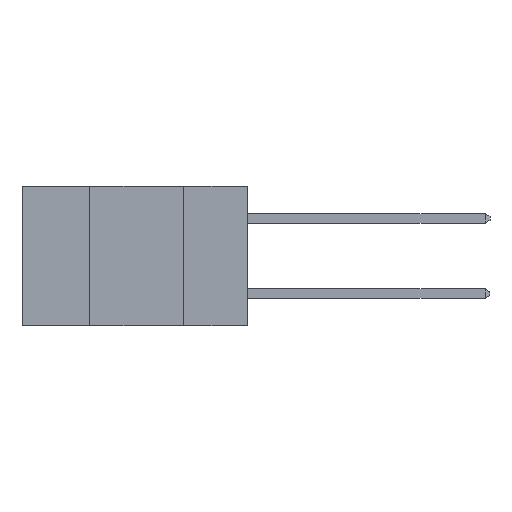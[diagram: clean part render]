
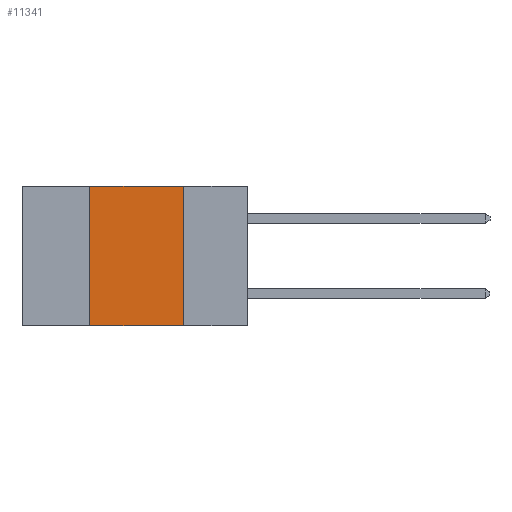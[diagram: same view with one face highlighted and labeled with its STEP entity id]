
A CAD part, left-side view. The second image highlights one B-rep face of the part: STEP entity #11341.
In plain terms, the highlighted planar face has unit normal (-1, 0, 0).
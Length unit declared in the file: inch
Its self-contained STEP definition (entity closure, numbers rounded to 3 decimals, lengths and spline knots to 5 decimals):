
#342 = VECTOR ( 'NONE', #9666, 39.37008 ) ;
#1164 = CARTESIAN_POINT ( 'NONE',  ( 0., 0.42, 0. ) ) ;
#1692 = CARTESIAN_POINT ( 'NONE',  ( 0., 0.6, -0.37 ) ) ;
#2035 = ORIENTED_EDGE ( 'NONE', *, *, #3957, .F. ) ;
#2105 = ORIENTED_EDGE ( 'NONE', *, *, #18469, .F. ) ;
#2183 = CARTESIAN_POINT ( 'NONE',  ( 0., 0.42, -0.37 ) ) ;
#2289 = LINE ( 'NONE', #7527, #10211 ) ;
#2621 = CARTESIAN_POINT ( 'NONE',  ( 0., 0.42, 0. ) ) ;
#2754 = ORIENTED_EDGE ( 'NONE', *, *, #2788, .F. ) ;
#2788 = EDGE_CURVE ( 'NONE', #3424, #3328, #13982, .T. ) ;
#3208 = CARTESIAN_POINT ( 'NONE',  ( 0., 0.6, 0. ) ) ;
#3328 = VERTEX_POINT ( 'NONE', #1164 ) ;
#3424 = VERTEX_POINT ( 'NONE', #2183 ) ;
#3551 = ORIENTED_EDGE ( 'NONE', *, *, #16769, .T. ) ;
#3810 = CARTESIAN_POINT ( 'NONE',  ( 0., 0.6, 0. ) ) ;
#3957 = EDGE_CURVE ( 'NONE', #9337, #6340, #2289, .T. ) ;
#4286 = DIRECTION ( 'NONE',  ( 0., 0., 1. ) ) ;
#4524 = FACE_OUTER_BOUND ( 'NONE', #12773, .T. ) ;
#4697 = LINE ( 'NONE', #1692, #342 ) ;
#4825 = DIRECTION ( 'NONE',  ( 0., 0., -1. ) ) ;
#5409 = VECTOR ( 'NONE', #4286, 39.37008 ) ;
#6340 = VERTEX_POINT ( 'NONE', #8010 ) ;
#7527 = CARTESIAN_POINT ( 'NONE',  ( 0., 0.17, 0. ) ) ;
#7822 = VECTOR ( 'NONE', #14526, 39.37008 ) ;
#8010 = CARTESIAN_POINT ( 'NONE',  ( 0., 0.17, -0.37 ) ) ;
#9337 = VERTEX_POINT ( 'NONE', #16933 ) ;
#9666 = DIRECTION ( 'NONE',  ( 0., -1., 0. ) ) ;
#10138 = AXIS2_PLACEMENT_3D ( 'NONE', #3208, #13976, #4825 ) ;
#10211 = VECTOR ( 'NONE', #10621, 39.37008 ) ;
#10621 = DIRECTION ( 'NONE',  ( 0., 0., -1. ) ) ;
#11010 = PLANE ( 'NONE',  #10138 ) ;
#11341 = ADVANCED_FACE ( 'NONE', ( #4524 ), #11010, .F. ) ;
#11414 = LINE ( 'NONE', #3810, #7822 ) ;
#12773 = EDGE_LOOP ( 'NONE', ( #2035, #2105, #2754, #3551 ) ) ;
#13976 = DIRECTION ( 'NONE',  ( 1., 0., 0. ) ) ;
#13982 = LINE ( 'NONE', #2621, #5409 ) ;
#14526 = DIRECTION ( 'NONE',  ( 0., -1., 0. ) ) ;
#16769 = EDGE_CURVE ( 'NONE', #3424, #6340, #4697, .T. ) ;
#16933 = CARTESIAN_POINT ( 'NONE',  ( 0., 0.17, 0. ) ) ;
#18469 = EDGE_CURVE ( 'NONE', #3328, #9337, #11414, .T. ) ;
